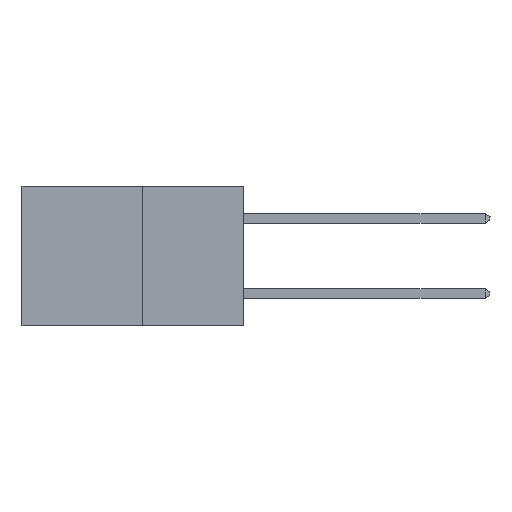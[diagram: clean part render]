
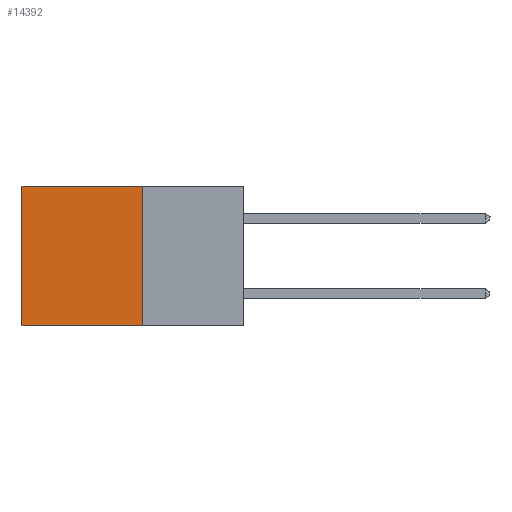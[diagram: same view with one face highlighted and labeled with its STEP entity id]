
A CAD part, left-side view. The second image highlights one B-rep face of the part: STEP entity #14392.
In plain terms, the highlighted planar face has unit normal (-1, 0, 0).
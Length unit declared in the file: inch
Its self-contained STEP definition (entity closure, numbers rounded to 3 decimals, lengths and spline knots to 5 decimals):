
#1174 = DIRECTION ( 'NONE',  ( 0., 1., 0. ) ) ;
#1208 = CARTESIAN_POINT ( 'NONE',  ( 0.277, 0.27, -0.37 ) ) ;
#2032 = EDGE_CURVE ( 'NONE', #12501, #15651, #8745, .T. ) ;
#3470 = CARTESIAN_POINT ( 'NONE',  ( 0.277, 0.27, -0.37 ) ) ;
#3891 = DIRECTION ( 'NONE',  ( 0., 1., 0. ) ) ;
#4163 = AXIS2_PLACEMENT_3D ( 'NONE', #3470, #4800, #13830 ) ;
#4532 = EDGE_LOOP ( 'NONE', ( #16365, #15350, #10236, #12141 ) ) ;
#4800 = DIRECTION ( 'NONE',  ( 1., 0., 0. ) ) ;
#4855 = CARTESIAN_POINT ( 'NONE',  ( 0.277, 0.59, 0. ) ) ;
#4902 = VECTOR ( 'NONE', #13072, 39.37008 ) ;
#6486 = CARTESIAN_POINT ( 'NONE',  ( 0.277, 0.27, 0. ) ) ;
#7558 = LINE ( 'NONE', #1208, #11748 ) ;
#8424 = EDGE_CURVE ( 'NONE', #15277, #15651, #16391, .T. ) ;
#8745 = LINE ( 'NONE', #15477, #4902 ) ;
#8815 = CARTESIAN_POINT ( 'NONE',  ( 0.277, 0.27, 0. ) ) ;
#8924 = CARTESIAN_POINT ( 'NONE',  ( 0.277, 0.27, -0.37 ) ) ;
#9569 = VERTEX_POINT ( 'NONE', #8815 ) ;
#9675 = CARTESIAN_POINT ( 'NONE',  ( 0.277, 0.27, -0.37 ) ) ;
#10236 = ORIENTED_EDGE ( 'NONE', *, *, #13205, .F. ) ;
#10286 = DIRECTION ( 'NONE',  ( 0., 0., -1. ) ) ;
#10961 = LINE ( 'NONE', #6486, #14000 ) ;
#11226 = PLANE ( 'NONE',  #4163 ) ;
#11748 = VECTOR ( 'NONE', #10286, 39.37008 ) ;
#12141 = ORIENTED_EDGE ( 'NONE', *, *, #13260, .T. ) ;
#12501 = VERTEX_POINT ( 'NONE', #4855 ) ;
#12941 = CARTESIAN_POINT ( 'NONE',  ( 0.277, 0.59, -0.37 ) ) ;
#12944 = VECTOR ( 'NONE', #1174, 39.37008 ) ;
#13072 = DIRECTION ( 'NONE',  ( 0., 0., -1. ) ) ;
#13205 = EDGE_CURVE ( 'NONE', #9569, #15277, #7558, .T. ) ;
#13260 = EDGE_CURVE ( 'NONE', #9569, #12501, #10961, .T. ) ;
#13830 = DIRECTION ( 'NONE',  ( 0., 0., -1. ) ) ;
#14000 = VECTOR ( 'NONE', #3891, 39.37008 ) ;
#14392 = ADVANCED_FACE ( 'NONE', ( #14601 ), #11226, .F. ) ;
#14601 = FACE_OUTER_BOUND ( 'NONE', #4532, .T. ) ;
#15277 = VERTEX_POINT ( 'NONE', #9675 ) ;
#15350 = ORIENTED_EDGE ( 'NONE', *, *, #8424, .F. ) ;
#15477 = CARTESIAN_POINT ( 'NONE',  ( 0.277, 0.59, -0.37 ) ) ;
#15651 = VERTEX_POINT ( 'NONE', #12941 ) ;
#16365 = ORIENTED_EDGE ( 'NONE', *, *, #2032, .T. ) ;
#16391 = LINE ( 'NONE', #8924, #12944 ) ;
